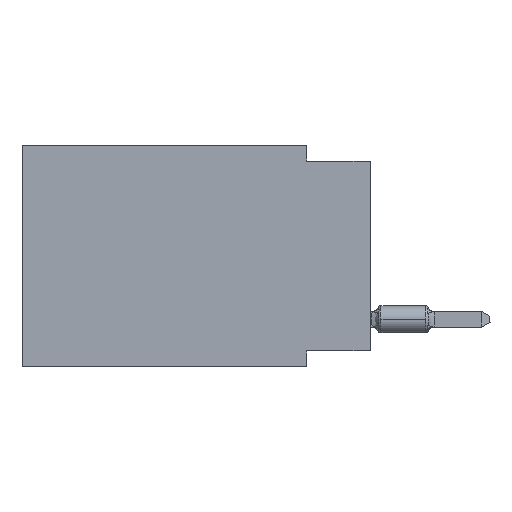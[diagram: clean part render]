
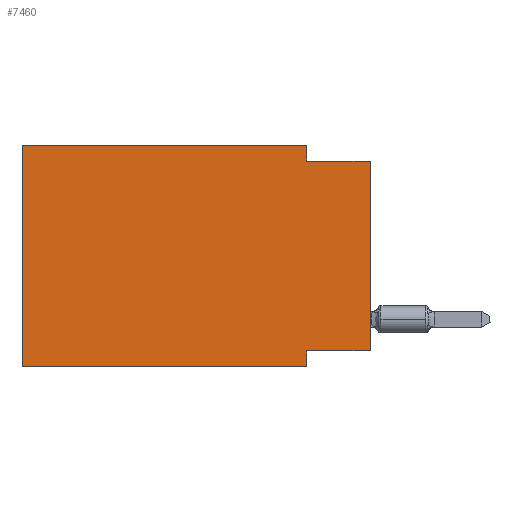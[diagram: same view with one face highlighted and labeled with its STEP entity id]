
A CAD part, left-side view. The second image highlights one B-rep face of the part: STEP entity #7460.
In plain terms, the highlighted planar face has unit normal (-1, 0, 0).
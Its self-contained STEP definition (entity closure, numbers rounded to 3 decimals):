
#124 = LINE ( 'NONE', #37826, #39380 ) ;
#934 = CARTESIAN_POINT ( 'NONE',  ( 0., 0., -0.635 ) ) ;
#2374 = EDGE_CURVE ( 'NONE', #29544, #12893, #43581, .T. ) ;
#2791 = CARTESIAN_POINT ( 'NONE',  ( 0., 13.97, 0. ) ) ;
#3289 = VERTEX_POINT ( 'NONE', #30282 ) ;
#4257 = CARTESIAN_POINT ( 'NONE',  ( 0., 2.54, -0.635 ) ) ;
#4381 = EDGE_LOOP ( 'NONE', ( #7514, #26972, #47796, #35689, #41716, #28846, #30409, #40846 ) ) ;
#4385 = VERTEX_POINT ( 'NONE', #2791 ) ;
#7119 = EDGE_CURVE ( 'NONE', #34566, #26688, #124, .T. ) ;
#7460 = ADVANCED_FACE ( 'NONE', ( #13999 ), #29089, .F. ) ;
#7514 = ORIENTED_EDGE ( 'NONE', *, *, #38607, .T. ) ;
#10388 = CARTESIAN_POINT ( 'NONE',  ( 0., 2.54, 0. ) ) ;
#11175 = VECTOR ( 'NONE', #21550, 1000. ) ;
#12357 = LINE ( 'NONE', #934, #39329 ) ;
#12893 = VERTEX_POINT ( 'NONE', #4257 ) ;
#13627 = EDGE_CURVE ( 'NONE', #3289, #23575, #30127, .T. ) ;
#13999 = FACE_OUTER_BOUND ( 'NONE', #4381, .T. ) ;
#14888 = LINE ( 'NONE', #45585, #42281 ) ;
#17954 = EDGE_CURVE ( 'NONE', #34566, #4385, #14888, .T. ) ;
#18007 = CARTESIAN_POINT ( 'NONE',  ( 0., 0., -8.255 ) ) ;
#18728 = VECTOR ( 'NONE', #32108, 1000. ) ;
#18896 = EDGE_CURVE ( 'NONE', #23575, #26688, #45911, .T. ) ;
#19419 = VERTEX_POINT ( 'NONE', #39831 ) ;
#20765 = CARTESIAN_POINT ( 'NONE',  ( 0., 2.54, -8.89 ) ) ;
#20963 = LINE ( 'NONE', #39310, #18728 ) ;
#21550 = DIRECTION ( 'NONE',  ( 0., 0., -1. ) ) ;
#23575 = VERTEX_POINT ( 'NONE', #42630 ) ;
#26688 = VERTEX_POINT ( 'NONE', #20765 ) ;
#26972 = ORIENTED_EDGE ( 'NONE', *, *, #31883, .F. ) ;
#28591 = DIRECTION ( 'NONE',  ( 1., 0., 0. ) ) ;
#28846 = ORIENTED_EDGE ( 'NONE', *, *, #7119, .T. ) ;
#28917 = LINE ( 'NONE', #40811, #30050 ) ;
#29089 = PLANE ( 'NONE',  #39279 ) ;
#29544 = VERTEX_POINT ( 'NONE', #39505 ) ;
#29808 = EDGE_CURVE ( 'NONE', #4385, #29544, #20963, .T. ) ;
#30050 = VECTOR ( 'NONE', #47992, 1000. ) ;
#30127 = LINE ( 'NONE', #18007, #45961 ) ;
#30282 = CARTESIAN_POINT ( 'NONE',  ( 0., 0., -8.255 ) ) ;
#30409 = ORIENTED_EDGE ( 'NONE', *, *, #18896, .F. ) ;
#31883 = EDGE_CURVE ( 'NONE', #12893, #19419, #12357, .T. ) ;
#32108 = DIRECTION ( 'NONE',  ( 0., -1., 0. ) ) ;
#34536 = DIRECTION ( 'NONE',  ( 0., 0., -1. ) ) ;
#34566 = VERTEX_POINT ( 'NONE', #36442 ) ;
#34772 = CARTESIAN_POINT ( 'NONE',  ( 0., 2.54, -8.89 ) ) ;
#35689 = ORIENTED_EDGE ( 'NONE', *, *, #29808, .F. ) ;
#36040 = DIRECTION ( 'NONE',  ( 0., 0., -1. ) ) ;
#36442 = CARTESIAN_POINT ( 'NONE',  ( 0., 13.97, -8.89 ) ) ;
#37577 = DIRECTION ( 'NONE',  ( 0., 1., 0. ) ) ;
#37582 = DIRECTION ( 'NONE',  ( 0., -1., 0. ) ) ;
#37826 = CARTESIAN_POINT ( 'NONE',  ( 0., 13.97, -8.89 ) ) ;
#38607 = EDGE_CURVE ( 'NONE', #3289, #19419, #28917, .T. ) ;
#39279 = AXIS2_PLACEMENT_3D ( 'NONE', #44193, #28591, #36040 ) ;
#39310 = CARTESIAN_POINT ( 'NONE',  ( 0., 13.97, 0. ) ) ;
#39329 = VECTOR ( 'NONE', #46536, 1000. ) ;
#39380 = VECTOR ( 'NONE', #37582, 1000. ) ;
#39505 = CARTESIAN_POINT ( 'NONE',  ( 0., 2.54, 0. ) ) ;
#39831 = CARTESIAN_POINT ( 'NONE',  ( 0., 0., -0.635 ) ) ;
#40811 = CARTESIAN_POINT ( 'NONE',  ( 0., 0., 0. ) ) ;
#40846 = ORIENTED_EDGE ( 'NONE', *, *, #13627, .F. ) ;
#41135 = DIRECTION ( 'NONE',  ( 0., 0., 1. ) ) ;
#41578 = VECTOR ( 'NONE', #34536, 1000. ) ;
#41716 = ORIENTED_EDGE ( 'NONE', *, *, #17954, .F. ) ;
#42281 = VECTOR ( 'NONE', #41135, 1000. ) ;
#42630 = CARTESIAN_POINT ( 'NONE',  ( 0., 2.54, -8.255 ) ) ;
#43581 = LINE ( 'NONE', #10388, #11175 ) ;
#44193 = CARTESIAN_POINT ( 'NONE',  ( 0., 13.97, 0. ) ) ;
#45585 = CARTESIAN_POINT ( 'NONE',  ( 0., 13.97, 0. ) ) ;
#45911 = LINE ( 'NONE', #34772, #41578 ) ;
#45961 = VECTOR ( 'NONE', #37577, 1000. ) ;
#46536 = DIRECTION ( 'NONE',  ( 0., -1., 0. ) ) ;
#47796 = ORIENTED_EDGE ( 'NONE', *, *, #2374, .F. ) ;
#47992 = DIRECTION ( 'NONE',  ( 0., 0., 1. ) ) ;
